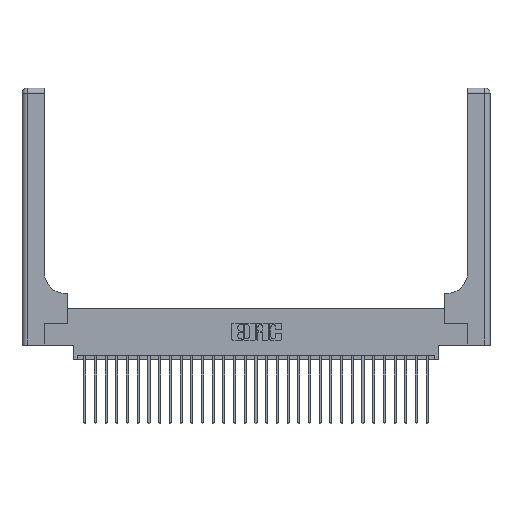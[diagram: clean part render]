
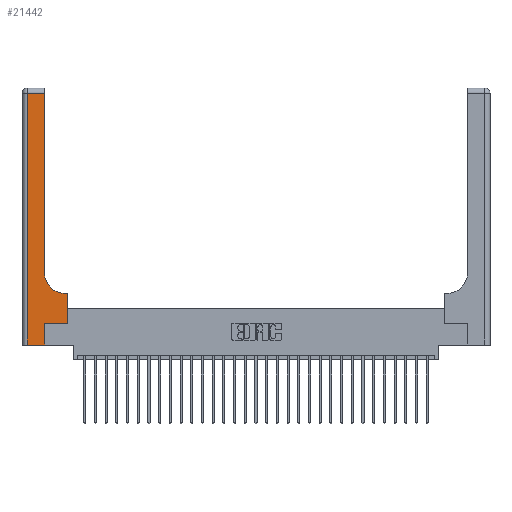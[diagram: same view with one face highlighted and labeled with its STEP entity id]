
A CAD part, top view. The second image highlights one B-rep face of the part: STEP entity #21442.
In plain terms, the highlighted planar face has unit normal (0, 0, 1).
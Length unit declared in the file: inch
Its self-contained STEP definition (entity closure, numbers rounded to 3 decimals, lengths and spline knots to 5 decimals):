
#17 = CARTESIAN_POINT ( 'NONE',  ( 0.528, 0.25, 0.37 ) ) ;
#1197 = LINE ( 'NONE', #1616, #25597 ) ;
#1596 = CIRCLE ( 'NONE', #17723, 0.25 ) ;
#1616 = CARTESIAN_POINT ( 'NONE',  ( 0.265, 0.25, 0.37 ) ) ;
#1724 = CARTESIAN_POINT ( 'NONE',  ( 0.26, 0.6, 0.37 ) ) ;
#1988 = ORIENTED_EDGE ( 'NONE', *, *, #23317, .T. ) ;
#1997 = CARTESIAN_POINT ( 'NONE',  ( 0.528, 0.6, 0.37 ) ) ;
#2125 = CARTESIAN_POINT ( 'NONE',  ( 0.265, 0., 0.37 ) ) ;
#2134 = EDGE_CURVE ( 'NONE', #7726, #7014, #11907, .T. ) ;
#2799 = ORIENTED_EDGE ( 'NONE', *, *, #18581, .T. ) ;
#3068 = PLANE ( 'NONE',  #10607 ) ;
#3367 = DIRECTION ( 'NONE',  ( 1., 0., 0. ) ) ;
#3566 = LINE ( 'NONE', #21569, #11889 ) ;
#3756 = LINE ( 'NONE', #1724, #21700 ) ;
#5229 = EDGE_LOOP ( 'NONE', ( #21024, #5352, #18032, #27160, #2799, #18821, #9751, #1988, #23496 ) ) ;
#5352 = ORIENTED_EDGE ( 'NONE', *, *, #16158, .T. ) ;
#5812 = CARTESIAN_POINT ( 'NONE',  ( 0., 3., 0.37 ) ) ;
#6807 = DIRECTION ( 'NONE',  ( 0., 1., 0. ) ) ;
#6818 = CARTESIAN_POINT ( 'NONE',  ( 0.06, 0., 0.37 ) ) ;
#7014 = VERTEX_POINT ( 'NONE', #27644 ) ;
#7648 = EDGE_CURVE ( 'NONE', #21701, #17108, #20039, .T. ) ;
#7693 = FACE_OUTER_BOUND ( 'NONE', #5229, .T. ) ;
#7726 = VERTEX_POINT ( 'NONE', #19763 ) ;
#7970 = DIRECTION ( 'NONE',  ( -1., 0., 0. ) ) ;
#8398 = LINE ( 'NONE', #17192, #23366 ) ;
#8820 = EDGE_CURVE ( 'NONE', #15372, #25419, #1197, .T. ) ;
#9226 = DIRECTION ( 'NONE',  ( 1., 0., 0. ) ) ;
#9751 = ORIENTED_EDGE ( 'NONE', *, *, #10793, .T. ) ;
#9807 = VECTOR ( 'NONE', #9226, 39.37008 ) ;
#9942 = CARTESIAN_POINT ( 'NONE',  ( 0.06, 2.94, 0.37 ) ) ;
#10607 = AXIS2_PLACEMENT_3D ( 'NONE', #5812, #27311, #7970 ) ;
#10793 = EDGE_CURVE ( 'NONE', #25419, #11735, #21918, .T. ) ;
#11284 = EDGE_CURVE ( 'NONE', #15642, #21701, #21784, .T. ) ;
#11735 = VERTEX_POINT ( 'NONE', #1997 ) ;
#11889 = VECTOR ( 'NONE', #14956, 39.37008 ) ;
#11907 = LINE ( 'NONE', #20394, #26861 ) ;
#13692 = EDGE_CURVE ( 'NONE', #15339, #7726, #1596, .T. ) ;
#14956 = DIRECTION ( 'NONE',  ( 0., 1., 0. ) ) ;
#15339 = VERTEX_POINT ( 'NONE', #21904 ) ;
#15372 = VERTEX_POINT ( 'NONE', #20458 ) ;
#15642 = VERTEX_POINT ( 'NONE', #9942 ) ;
#15857 = CARTESIAN_POINT ( 'NONE',  ( 0., 0., 0.37 ) ) ;
#16158 = EDGE_CURVE ( 'NONE', #7014, #15642, #8398, .T. ) ;
#17016 = DIRECTION ( 'NONE',  ( -1., 0., 0. ) ) ;
#17108 = VERTEX_POINT ( 'NONE', #2125 ) ;
#17192 = CARTESIAN_POINT ( 'NONE',  ( 0., 2.94, 0.37 ) ) ;
#17723 = AXIS2_PLACEMENT_3D ( 'NONE', #18554, #20723, #24770 ) ;
#18032 = ORIENTED_EDGE ( 'NONE', *, *, #11284, .T. ) ;
#18386 = DIRECTION ( 'NONE',  ( 0., 1., 0. ) ) ;
#18554 = CARTESIAN_POINT ( 'NONE',  ( 0.51, 0.85, 0.37 ) ) ;
#18581 = EDGE_CURVE ( 'NONE', #17108, #15372, #3566, .T. ) ;
#18821 = ORIENTED_EDGE ( 'NONE', *, *, #8820, .T. ) ;
#19625 = CARTESIAN_POINT ( 'NONE',  ( 0.528, 0.25, 0.37 ) ) ;
#19763 = CARTESIAN_POINT ( 'NONE',  ( 0.26, 0.85, 0.37 ) ) ;
#20039 = LINE ( 'NONE', #15857, #9807 ) ;
#20394 = CARTESIAN_POINT ( 'NONE',  ( 0.26, 3., 0.37 ) ) ;
#20402 = VECTOR ( 'NONE', #26717, 39.37008 ) ;
#20458 = CARTESIAN_POINT ( 'NONE',  ( 0.265, 0.25, 0.37 ) ) ;
#20723 = DIRECTION ( 'NONE',  ( 0., 0., -1. ) ) ;
#21024 = ORIENTED_EDGE ( 'NONE', *, *, #2134, .T. ) ;
#21442 = ADVANCED_FACE ( 'NONE', ( #7693 ), #3068, .F. ) ;
#21569 = CARTESIAN_POINT ( 'NONE',  ( 0.265, 0., 0.37 ) ) ;
#21700 = VECTOR ( 'NONE', #17016, 39.37008 ) ;
#21701 = VERTEX_POINT ( 'NONE', #6818 ) ;
#21784 = LINE ( 'NONE', #28463, #20402 ) ;
#21904 = CARTESIAN_POINT ( 'NONE',  ( 0.51, 0.6, 0.37 ) ) ;
#21918 = LINE ( 'NONE', #19625, #22227 ) ;
#22227 = VECTOR ( 'NONE', #6807, 39.37008 ) ;
#23317 = EDGE_CURVE ( 'NONE', #11735, #15339, #3756, .T. ) ;
#23366 = VECTOR ( 'NONE', #25995, 39.37008 ) ;
#23496 = ORIENTED_EDGE ( 'NONE', *, *, #13692, .T. ) ;
#24770 = DIRECTION ( 'NONE',  ( 1., 0., 0. ) ) ;
#25419 = VERTEX_POINT ( 'NONE', #17 ) ;
#25597 = VECTOR ( 'NONE', #3367, 39.37008 ) ;
#25995 = DIRECTION ( 'NONE',  ( -1., 0., 0. ) ) ;
#26717 = DIRECTION ( 'NONE',  ( 0., -1., 0. ) ) ;
#26861 = VECTOR ( 'NONE', #18386, 39.37008 ) ;
#27160 = ORIENTED_EDGE ( 'NONE', *, *, #7648, .T. ) ;
#27311 = DIRECTION ( 'NONE',  ( 0., 0., -1. ) ) ;
#27644 = CARTESIAN_POINT ( 'NONE',  ( 0.26, 2.94, 0.37 ) ) ;
#28463 = CARTESIAN_POINT ( 'NONE',  ( 0.06, 3., 0.37 ) ) ;
